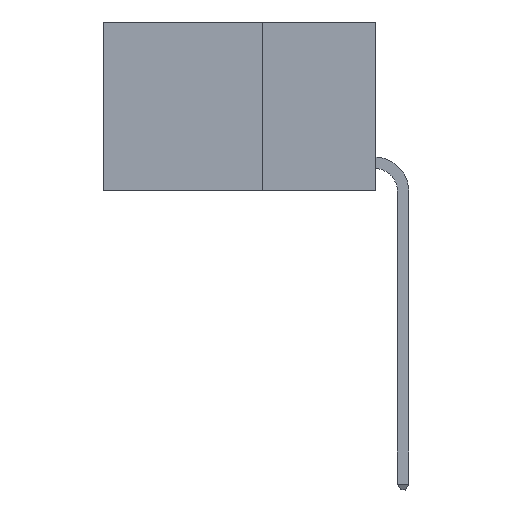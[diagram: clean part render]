
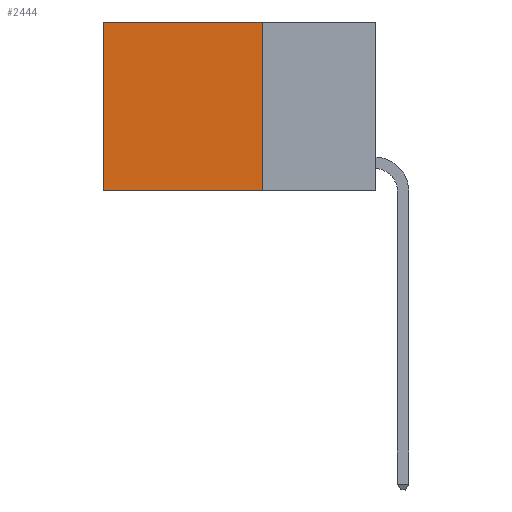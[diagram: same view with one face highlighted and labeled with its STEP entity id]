
A CAD part, left-side view. The second image highlights one B-rep face of the part: STEP entity #2444.
In plain terms, the highlighted planar face has unit normal (-1, 0, 0).
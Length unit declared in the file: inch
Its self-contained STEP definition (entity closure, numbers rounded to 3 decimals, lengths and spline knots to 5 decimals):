
#669 = DIRECTION ( 'NONE',  ( 0., 0., -1. ) ) ;
#893 = CARTESIAN_POINT ( 'NONE',  ( 0.2625, 0.25, -0.37 ) ) ;
#2177 = CARTESIAN_POINT ( 'NONE',  ( 0.2625, 0.25, 0. ) ) ;
#2254 = VECTOR ( 'NONE', #10344, 39.37008 ) ;
#2436 = LINE ( 'NONE', #18459, #7851 ) ;
#2444 = ADVANCED_FACE ( 'NONE', ( #17048 ), #12727, .F. ) ;
#2952 = DIRECTION ( 'NONE',  ( 0., 1., 0. ) ) ;
#3687 = ORIENTED_EDGE ( 'NONE', *, *, #10330, .F. ) ;
#4044 = LINE ( 'NONE', #6846, #24257 ) ;
#5947 = VECTOR ( 'NONE', #2952, 39.37008 ) ;
#6250 = VERTEX_POINT ( 'NONE', #12667 ) ;
#6405 = DIRECTION ( 'NONE',  ( 0., 0., -1. ) ) ;
#6703 = CARTESIAN_POINT ( 'NONE',  ( 0.2625, 0.25, -0.37 ) ) ;
#6846 = CARTESIAN_POINT ( 'NONE',  ( 0.2625, 0.25, 0. ) ) ;
#7473 = EDGE_CURVE ( 'NONE', #16766, #6250, #23755, .T. ) ;
#7851 = VECTOR ( 'NONE', #6405, 39.37008 ) ;
#8261 = VERTEX_POINT ( 'NONE', #6703 ) ;
#9348 = ORIENTED_EDGE ( 'NONE', *, *, #15087, .T. ) ;
#9622 = EDGE_CURVE ( 'NONE', #16766, #8261, #4044, .T. ) ;
#10330 = EDGE_CURVE ( 'NONE', #8261, #22115, #22019, .T. ) ;
#10344 = DIRECTION ( 'NONE',  ( 0., 1., 0. ) ) ;
#11905 = AXIS2_PLACEMENT_3D ( 'NONE', #22893, #12817, #669 ) ;
#12667 = CARTESIAN_POINT ( 'NONE',  ( 0.2625, 0.6, 0. ) ) ;
#12717 = EDGE_LOOP ( 'NONE', ( #9348, #3687, #22604, #16670 ) ) ;
#12727 = PLANE ( 'NONE',  #11905 ) ;
#12817 = DIRECTION ( 'NONE',  ( 1., 0., 0. ) ) ;
#13298 = CARTESIAN_POINT ( 'NONE',  ( 0.2625, 0.6, -0.37 ) ) ;
#15087 = EDGE_CURVE ( 'NONE', #6250, #22115, #2436, .T. ) ;
#16670 = ORIENTED_EDGE ( 'NONE', *, *, #7473, .T. ) ;
#16766 = VERTEX_POINT ( 'NONE', #25906 ) ;
#17048 = FACE_OUTER_BOUND ( 'NONE', #12717, .T. ) ;
#18459 = CARTESIAN_POINT ( 'NONE',  ( 0.2625, 0.6, 0. ) ) ;
#22019 = LINE ( 'NONE', #893, #5947 ) ;
#22115 = VERTEX_POINT ( 'NONE', #13298 ) ;
#22604 = ORIENTED_EDGE ( 'NONE', *, *, #9622, .F. ) ;
#22893 = CARTESIAN_POINT ( 'NONE',  ( 0.2625, 0.25, 0. ) ) ;
#23755 = LINE ( 'NONE', #2177, #2254 ) ;
#24257 = VECTOR ( 'NONE', #24866, 39.37008 ) ;
#24866 = DIRECTION ( 'NONE',  ( 0., 0., -1. ) ) ;
#25906 = CARTESIAN_POINT ( 'NONE',  ( 0.2625, 0.25, 0. ) ) ;
